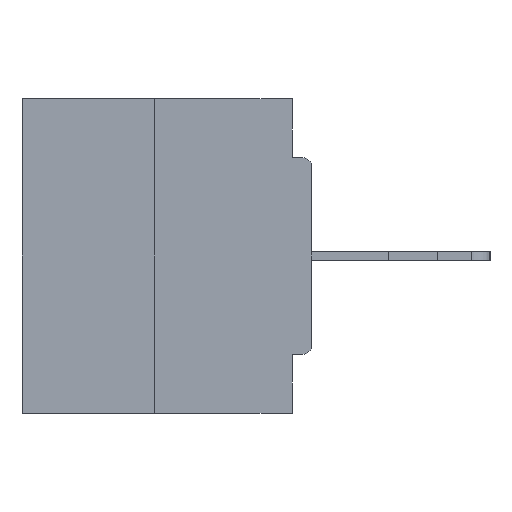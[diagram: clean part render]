
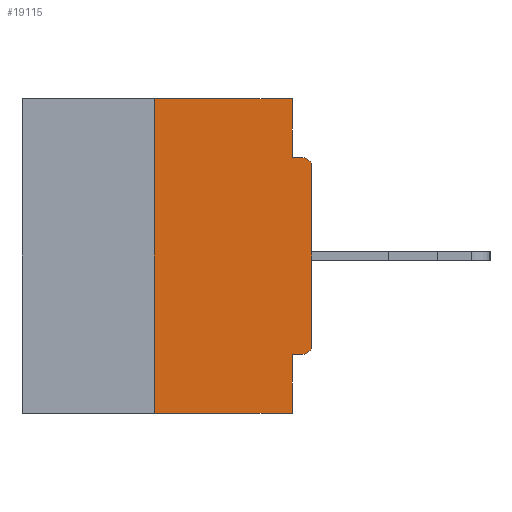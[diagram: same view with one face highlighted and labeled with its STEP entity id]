
A CAD part, left-side view. The second image highlights one B-rep face of the part: STEP entity #19115.
In plain terms, the highlighted planar face has unit normal (-1, 0, 0).
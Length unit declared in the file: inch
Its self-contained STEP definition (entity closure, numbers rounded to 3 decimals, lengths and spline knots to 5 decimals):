
#472 = VECTOR ( 'NONE', #23473, 39.37008 ) ;
#494 = CARTESIAN_POINT ( 'NONE',  ( 0., 0.25, -0.5 ) ) ;
#1831 = VERTEX_POINT ( 'NONE', #5355 ) ;
#1901 = AXIS2_PLACEMENT_3D ( 'NONE', #15775, #27596, #11949 ) ;
#2500 = ORIENTED_EDGE ( 'NONE', *, *, #37203, .T. ) ;
#3548 = VERTEX_POINT ( 'NONE', #29869 ) ;
#3561 = DIRECTION ( 'NONE',  ( 0., -1., 0. ) ) ;
#3843 = CIRCLE ( 'NONE', #1901, 0.015 ) ;
#5355 = CARTESIAN_POINT ( 'NONE',  ( 0., 0.031, 0. ) ) ;
#5830 = AXIS2_PLACEMENT_3D ( 'NONE', #23930, #39193, #11151 ) ;
#6056 = DIRECTION ( 'NONE',  ( 0., 0., -1. ) ) ;
#6079 = VERTEX_POINT ( 'NONE', #33298 ) ;
#6085 = CARTESIAN_POINT ( 'NONE',  ( 0., 0.031, -0.0935 ) ) ;
#7193 = VERTEX_POINT ( 'NONE', #32678 ) ;
#8157 = DIRECTION ( 'NONE',  ( 0., 0., -1. ) ) ;
#8424 = EDGE_CURVE ( 'NONE', #6079, #37380, #13719, .T. ) ;
#8935 = CARTESIAN_POINT ( 'NONE',  ( 0., 0., -0.0935 ) ) ;
#9067 = VERTEX_POINT ( 'NONE', #494 ) ;
#9074 = CIRCLE ( 'NONE', #5830, 0.015 ) ;
#9105 = CARTESIAN_POINT ( 'NONE',  ( 0., 0.46, -0.5 ) ) ;
#9268 = ORIENTED_EDGE ( 'NONE', *, *, #24334, .F. ) ;
#9567 = CARTESIAN_POINT ( 'NONE',  ( 0., 0.25, 0. ) ) ;
#11151 = DIRECTION ( 'NONE',  ( 0., 0., -1. ) ) ;
#11591 = LINE ( 'NONE', #17264, #17268 ) ;
#11895 = DIRECTION ( 'NONE',  ( 1., 0., 0. ) ) ;
#11949 = DIRECTION ( 'NONE',  ( 0., 0., -1. ) ) ;
#12084 = VERTEX_POINT ( 'NONE', #26394 ) ;
#12594 = ORIENTED_EDGE ( 'NONE', *, *, #38572, .F. ) ;
#13719 = LINE ( 'NONE', #14131, #472 ) ;
#14131 = CARTESIAN_POINT ( 'NONE',  ( 0., 0., -0.4065 ) ) ;
#14219 = VECTOR ( 'NONE', #23728, 39.37008 ) ;
#15673 = EDGE_CURVE ( 'NONE', #16391, #12084, #3843, .T. ) ;
#15775 = CARTESIAN_POINT ( 'NONE',  ( 0., 0.015, -0.1085 ) ) ;
#15883 = EDGE_LOOP ( 'NONE', ( #39798, #9268, #35623, #32588, #37023, #2500, #38971, #30045, #12594, #37814 ) ) ;
#16391 = VERTEX_POINT ( 'NONE', #23066 ) ;
#17264 = CARTESIAN_POINT ( 'NONE',  ( 0., 0.031, -0.5 ) ) ;
#17268 = VECTOR ( 'NONE', #8157, 39.37008 ) ;
#18019 = DIRECTION ( 'NONE',  ( 0., -1., 0. ) ) ;
#18318 = CARTESIAN_POINT ( 'NONE',  ( 0., 0.25, 0. ) ) ;
#18382 = FACE_OUTER_BOUND ( 'NONE', #15883, .T. ) ;
#18766 = CARTESIAN_POINT ( 'NONE',  ( 0., 0.46, 0. ) ) ;
#19071 = LINE ( 'NONE', #9567, #21809 ) ;
#19115 = ADVANCED_FACE ( 'NONE', ( #18382 ), #27534, .F. ) ;
#21809 = VECTOR ( 'NONE', #28427, 39.37008 ) ;
#22253 = EDGE_CURVE ( 'NONE', #40123, #1831, #25445, .T. ) ;
#22998 = VECTOR ( 'NONE', #18019, 39.37008 ) ;
#23066 = CARTESIAN_POINT ( 'NONE',  ( 0., 0., -0.1085 ) ) ;
#23365 = AXIS2_PLACEMENT_3D ( 'NONE', #33437, #11895, #24277 ) ;
#23473 = DIRECTION ( 'NONE',  ( 0., 1., 0. ) ) ;
#23532 = LINE ( 'NONE', #30443, #34787 ) ;
#23728 = DIRECTION ( 'NONE',  ( 0., -1., 0. ) ) ;
#23930 = CARTESIAN_POINT ( 'NONE',  ( 0., 0.015, -0.3915 ) ) ;
#24277 = DIRECTION ( 'NONE',  ( 0., 0., -1. ) ) ;
#24334 = EDGE_CURVE ( 'NONE', #9067, #40123, #19071, .T. ) ;
#24579 = EDGE_CURVE ( 'NONE', #7193, #16391, #23532, .T. ) ;
#25306 = CARTESIAN_POINT ( 'NONE',  ( 0., 0.031, 0. ) ) ;
#25445 = LINE ( 'NONE', #18766, #27510 ) ;
#26394 = CARTESIAN_POINT ( 'NONE',  ( 0., 0.015, -0.0935 ) ) ;
#26495 = EDGE_CURVE ( 'NONE', #1831, #30594, #33865, .T. ) ;
#27503 = EDGE_CURVE ( 'NONE', #37380, #3548, #11591, .T. ) ;
#27510 = VECTOR ( 'NONE', #3561, 39.37008 ) ;
#27534 = PLANE ( 'NONE',  #23365 ) ;
#27596 = DIRECTION ( 'NONE',  ( -1., 0., 0. ) ) ;
#28427 = DIRECTION ( 'NONE',  ( 0., 0., 1. ) ) ;
#29869 = CARTESIAN_POINT ( 'NONE',  ( 0., 0.031, -0.5 ) ) ;
#30045 = ORIENTED_EDGE ( 'NONE', *, *, #15673, .T. ) ;
#30443 = CARTESIAN_POINT ( 'NONE',  ( 0., 0., 0. ) ) ;
#30594 = VERTEX_POINT ( 'NONE', #6085 ) ;
#32588 = ORIENTED_EDGE ( 'NONE', *, *, #27503, .F. ) ;
#32658 = EDGE_CURVE ( 'NONE', #9067, #3548, #39966, .T. ) ;
#32678 = CARTESIAN_POINT ( 'NONE',  ( 0., 0., -0.3915 ) ) ;
#33088 = LINE ( 'NONE', #8935, #14219 ) ;
#33298 = CARTESIAN_POINT ( 'NONE',  ( 0., 0.015, -0.4065 ) ) ;
#33437 = CARTESIAN_POINT ( 'NONE',  ( 0., 0.46, 0. ) ) ;
#33696 = CARTESIAN_POINT ( 'NONE',  ( 0., 0.031, -0.4065 ) ) ;
#33865 = LINE ( 'NONE', #25306, #36669 ) ;
#34787 = VECTOR ( 'NONE', #35921, 39.37008 ) ;
#35623 = ORIENTED_EDGE ( 'NONE', *, *, #32658, .T. ) ;
#35921 = DIRECTION ( 'NONE',  ( 0., 0., 1. ) ) ;
#36669 = VECTOR ( 'NONE', #6056, 39.37008 ) ;
#37023 = ORIENTED_EDGE ( 'NONE', *, *, #8424, .F. ) ;
#37203 = EDGE_CURVE ( 'NONE', #6079, #7193, #9074, .T. ) ;
#37380 = VERTEX_POINT ( 'NONE', #33696 ) ;
#37814 = ORIENTED_EDGE ( 'NONE', *, *, #26495, .F. ) ;
#38572 = EDGE_CURVE ( 'NONE', #30594, #12084, #33088, .T. ) ;
#38971 = ORIENTED_EDGE ( 'NONE', *, *, #24579, .T. ) ;
#39193 = DIRECTION ( 'NONE',  ( -1., 0., 0. ) ) ;
#39798 = ORIENTED_EDGE ( 'NONE', *, *, #22253, .F. ) ;
#39966 = LINE ( 'NONE', #9105, #22998 ) ;
#40123 = VERTEX_POINT ( 'NONE', #18318 ) ;
